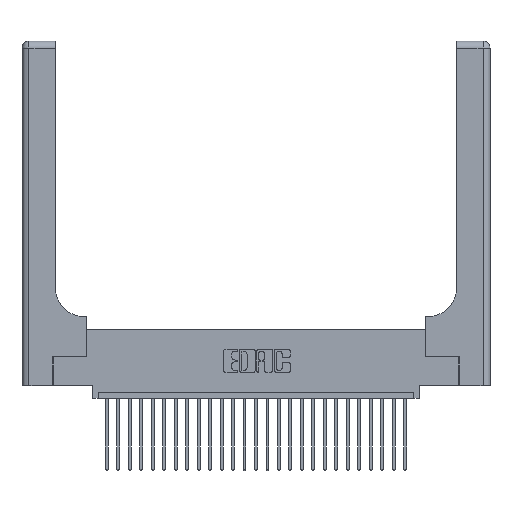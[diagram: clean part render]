
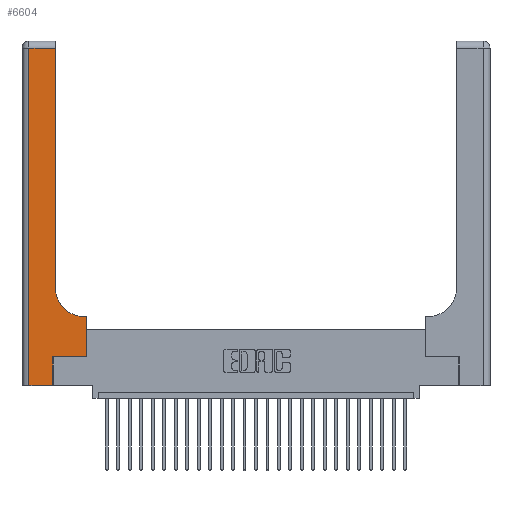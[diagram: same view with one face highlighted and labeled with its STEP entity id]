
A CAD part, top view. The second image highlights one B-rep face of the part: STEP entity #6604.
In plain terms, the highlighted planar face has unit normal (0, 0, 1).
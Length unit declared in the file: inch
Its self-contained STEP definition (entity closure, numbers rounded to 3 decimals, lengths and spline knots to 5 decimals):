
#798 = VECTOR ( 'NONE', #19935, 39.37008 ) ;
#1302 = CIRCLE ( 'NONE', #11126, 0.25 ) ;
#1726 = ORIENTED_EDGE ( 'NONE', *, *, #7093, .T. ) ;
#1753 = CARTESIAN_POINT ( 'NONE',  ( 0.2915, 0.85, 0.37 ) ) ;
#2096 = CARTESIAN_POINT ( 'NONE',  ( 0.2915, 2.94, 0.37 ) ) ;
#2328 = FACE_OUTER_BOUND ( 'NONE', #3527, .T. ) ;
#2372 = DIRECTION ( 'NONE',  ( 0., 1., 0. ) ) ;
#2470 = DIRECTION ( 'NONE',  ( 0., 0., -1. ) ) ;
#2950 = DIRECTION ( 'NONE',  ( 1., 0., 0. ) ) ;
#3231 = VERTEX_POINT ( 'NONE', #16400 ) ;
#3314 = VERTEX_POINT ( 'NONE', #19124 ) ;
#3379 = LINE ( 'NONE', #20102, #17462 ) ;
#3527 = EDGE_LOOP ( 'NONE', ( #6744, #10869, #11671, #1726, #14849, #11649, #17479, #9119, #22376 ) ) ;
#3539 = DIRECTION ( 'NONE',  ( -1., 0., 0. ) ) ;
#4203 = VERTEX_POINT ( 'NONE', #21468 ) ;
#5528 = VECTOR ( 'NONE', #3539, 39.37008 ) ;
#5618 = DIRECTION ( 'NONE',  ( 1., 0., 0. ) ) ;
#6345 = EDGE_CURVE ( 'NONE', #18766, #20175, #3379, .T. ) ;
#6552 = CARTESIAN_POINT ( 'NONE',  ( 0.269, 0.25, 0.37 ) ) ;
#6593 = EDGE_CURVE ( 'NONE', #3231, #4203, #26692, .T. ) ;
#6604 = ADVANCED_FACE ( 'NONE', ( #2328 ), #21624, .F. ) ;
#6744 = ORIENTED_EDGE ( 'NONE', *, *, #6345, .T. ) ;
#7011 = CARTESIAN_POINT ( 'NONE',  ( 0.06, 3., 0.37 ) ) ;
#7093 = EDGE_CURVE ( 'NONE', #3314, #21657, #17880, .T. ) ;
#7471 = DIRECTION ( 'NONE',  ( 0., -1., 0. ) ) ;
#7825 = VERTEX_POINT ( 'NONE', #6552 ) ;
#8051 = CARTESIAN_POINT ( 'NONE',  ( 0.269, 0., 0.37 ) ) ;
#8453 = LINE ( 'NONE', #7011, #17492 ) ;
#9119 = ORIENTED_EDGE ( 'NONE', *, *, #14489, .T. ) ;
#9557 = CARTESIAN_POINT ( 'NONE',  ( 0., 2.94, 0.37 ) ) ;
#9635 = EDGE_CURVE ( 'NONE', #20175, #18912, #26189, .T. ) ;
#9743 = LINE ( 'NONE', #24605, #5528 ) ;
#10546 = CARTESIAN_POINT ( 'NONE',  ( 0., 0., 0.37 ) ) ;
#10869 = ORIENTED_EDGE ( 'NONE', *, *, #9635, .T. ) ;
#11126 = AXIS2_PLACEMENT_3D ( 'NONE', #17757, #11331, #2950 ) ;
#11173 = VECTOR ( 'NONE', #5618, 39.37008 ) ;
#11331 = DIRECTION ( 'NONE',  ( 0., 0., -1. ) ) ;
#11649 = ORIENTED_EDGE ( 'NONE', *, *, #21287, .T. ) ;
#11671 = ORIENTED_EDGE ( 'NONE', *, *, #21717, .T. ) ;
#12859 = CARTESIAN_POINT ( 'NONE',  ( 0.5415, 0.6, 0.37 ) ) ;
#13363 = EDGE_CURVE ( 'NONE', #18988, #18766, #1302, .T. ) ;
#13692 = AXIS2_PLACEMENT_3D ( 'NONE', #21899, #2470, #21537 ) ;
#14489 = EDGE_CURVE ( 'NONE', #4203, #18988, #9743, .T. ) ;
#14849 = ORIENTED_EDGE ( 'NONE', *, *, #16001, .T. ) ;
#16001 = EDGE_CURVE ( 'NONE', #21657, #7825, #19377, .T. ) ;
#16329 = DIRECTION ( 'NONE',  ( 0., 1., 0. ) ) ;
#16400 = CARTESIAN_POINT ( 'NONE',  ( 0.5585, 0.25, 0.37 ) ) ;
#17462 = VECTOR ( 'NONE', #24141, 39.37008 ) ;
#17479 = ORIENTED_EDGE ( 'NONE', *, *, #6593, .T. ) ;
#17492 = VECTOR ( 'NONE', #7471, 39.37008 ) ;
#17757 = CARTESIAN_POINT ( 'NONE',  ( 0.5415, 0.85, 0.37 ) ) ;
#17880 = LINE ( 'NONE', #10546, #24152 ) ;
#18068 = CARTESIAN_POINT ( 'NONE',  ( 0.269, 0., 0.37 ) ) ;
#18766 = VERTEX_POINT ( 'NONE', #1753 ) ;
#18912 = VERTEX_POINT ( 'NONE', #27598 ) ;
#18988 = VERTEX_POINT ( 'NONE', #12859 ) ;
#19124 = CARTESIAN_POINT ( 'NONE',  ( 0.06, 0., 0.37 ) ) ;
#19377 = LINE ( 'NONE', #8051, #22003 ) ;
#19935 = DIRECTION ( 'NONE',  ( -1., 0., 0. ) ) ;
#20102 = CARTESIAN_POINT ( 'NONE',  ( 0.2915, 3., 0.37 ) ) ;
#20175 = VERTEX_POINT ( 'NONE', #2096 ) ;
#20769 = CARTESIAN_POINT ( 'NONE',  ( 0.269, 0.25, 0.37 ) ) ;
#21287 = EDGE_CURVE ( 'NONE', #7825, #3231, #21799, .T. ) ;
#21351 = CARTESIAN_POINT ( 'NONE',  ( 0.5585, 0.25, 0.37 ) ) ;
#21468 = CARTESIAN_POINT ( 'NONE',  ( 0.5585, 0.6, 0.37 ) ) ;
#21537 = DIRECTION ( 'NONE',  ( -1., 0., 0. ) ) ;
#21624 = PLANE ( 'NONE',  #13692 ) ;
#21657 = VERTEX_POINT ( 'NONE', #18068 ) ;
#21717 = EDGE_CURVE ( 'NONE', #18912, #3314, #8453, .T. ) ;
#21799 = LINE ( 'NONE', #20769, #11173 ) ;
#21899 = CARTESIAN_POINT ( 'NONE',  ( 0., 3., 0.37 ) ) ;
#22003 = VECTOR ( 'NONE', #16329, 39.37008 ) ;
#22376 = ORIENTED_EDGE ( 'NONE', *, *, #13363, .T. ) ;
#24141 = DIRECTION ( 'NONE',  ( 0., 1., 0. ) ) ;
#24152 = VECTOR ( 'NONE', #27364, 39.37008 ) ;
#24605 = CARTESIAN_POINT ( 'NONE',  ( 0.2915, 0.6, 0.37 ) ) ;
#26189 = LINE ( 'NONE', #9557, #798 ) ;
#26365 = VECTOR ( 'NONE', #2372, 39.37008 ) ;
#26692 = LINE ( 'NONE', #21351, #26365 ) ;
#27364 = DIRECTION ( 'NONE',  ( 1., 0., 0. ) ) ;
#27598 = CARTESIAN_POINT ( 'NONE',  ( 0.06, 2.94, 0.37 ) ) ;
